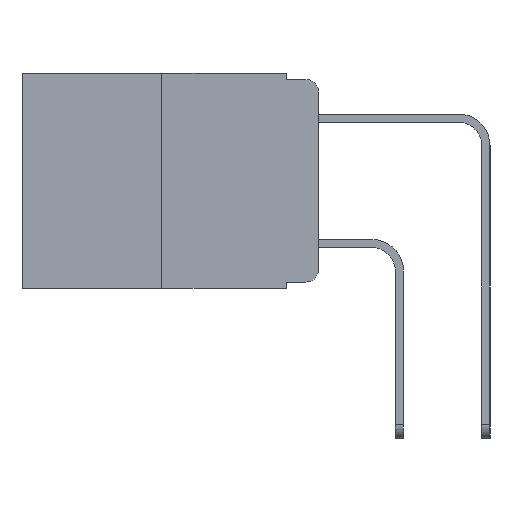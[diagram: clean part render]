
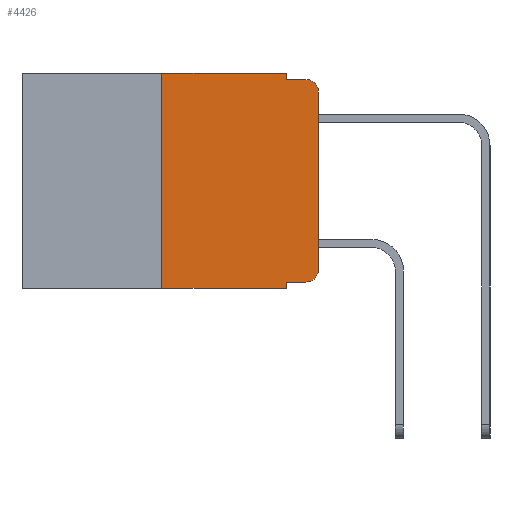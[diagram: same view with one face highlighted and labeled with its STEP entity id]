
A CAD part, left-side view. The second image highlights one B-rep face of the part: STEP entity #4426.
In plain terms, the highlighted planar face has unit normal (-1, 0, 0).
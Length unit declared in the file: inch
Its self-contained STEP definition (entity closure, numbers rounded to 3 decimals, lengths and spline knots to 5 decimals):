
#497 = DIRECTION ( 'NONE',  ( 0., -1., 0. ) ) ;
#598 = CARTESIAN_POINT ( 'NONE',  ( 0., 0.051, -0.333 ) ) ;
#1144 = DIRECTION ( 'NONE',  ( -1., 0., 0. ) ) ;
#1272 = VERTEX_POINT ( 'NONE', #2296 ) ;
#1951 = LINE ( 'NONE', #18520, #19803 ) ;
#2296 = CARTESIAN_POINT ( 'NONE',  ( 0., 0.051, 0. ) ) ;
#2344 = ORIENTED_EDGE ( 'NONE', *, *, #18447, .F. ) ;
#2579 = CARTESIAN_POINT ( 'NONE',  ( 0., 0., -0.313 ) ) ;
#2777 = VERTEX_POINT ( 'NONE', #12425 ) ;
#3322 = CARTESIAN_POINT ( 'NONE',  ( 0., 0.051, 0. ) ) ;
#3454 = CARTESIAN_POINT ( 'NONE',  ( 0., 0.02, -0.01 ) ) ;
#3554 = ORIENTED_EDGE ( 'NONE', *, *, #20716, .T. ) ;
#3621 = CARTESIAN_POINT ( 'NONE',  ( 0., 0.051, -0.333 ) ) ;
#3955 = ORIENTED_EDGE ( 'NONE', *, *, #10687, .F. ) ;
#4123 = CARTESIAN_POINT ( 'NONE',  ( 0., 0.473, -0.343 ) ) ;
#4220 = LINE ( 'NONE', #4123, #22340 ) ;
#4245 = DIRECTION ( 'NONE',  ( 0., 0., -1. ) ) ;
#4426 = ADVANCED_FACE ( 'NONE', ( #16488 ), #11996, .F. ) ;
#4604 = ORIENTED_EDGE ( 'NONE', *, *, #16158, .F. ) ;
#4806 = CARTESIAN_POINT ( 'NONE',  ( 0., 0.25, 0. ) ) ;
#4934 = ORIENTED_EDGE ( 'NONE', *, *, #22171, .T. ) ;
#5609 = ORIENTED_EDGE ( 'NONE', *, *, #14974, .F. ) ;
#5926 = CARTESIAN_POINT ( 'NONE',  ( 0., 0.051, -0.01 ) ) ;
#5939 = CARTESIAN_POINT ( 'NONE',  ( 0., 0., 0. ) ) ;
#5958 = DIRECTION ( 'NONE',  ( 0., -1., 0. ) ) ;
#6283 = VERTEX_POINT ( 'NONE', #3454 ) ;
#6377 = AXIS2_PLACEMENT_3D ( 'NONE', #12093, #1144, #13879 ) ;
#6570 = VERTEX_POINT ( 'NONE', #598 ) ;
#6986 = CARTESIAN_POINT ( 'NONE',  ( 0., 0.25, -0.343 ) ) ;
#7050 = CARTESIAN_POINT ( 'NONE',  ( 0., 0.473, 0. ) ) ;
#7569 = ORIENTED_EDGE ( 'NONE', *, *, #11403, .T. ) ;
#8119 = VECTOR ( 'NONE', #497, 39.37008 ) ;
#8121 = LINE ( 'NONE', #3322, #12861 ) ;
#8598 = CARTESIAN_POINT ( 'NONE',  ( 0., 0.051, -0.01 ) ) ;
#8909 = CARTESIAN_POINT ( 'NONE',  ( 0., 0.051, -0.343 ) ) ;
#10311 = DIRECTION ( 'NONE',  ( 0., 0., 1. ) ) ;
#10410 = LINE ( 'NONE', #3621, #14578 ) ;
#10466 = CARTESIAN_POINT ( 'NONE',  ( 0., 0.473, 0. ) ) ;
#10571 = VERTEX_POINT ( 'NONE', #8598 ) ;
#10687 = EDGE_CURVE ( 'NONE', #18016, #1272, #12916, .T. ) ;
#10804 = CARTESIAN_POINT ( 'NONE',  ( 0., 0.02, -0.313 ) ) ;
#11403 = EDGE_CURVE ( 'NONE', #2777, #19017, #22267, .T. ) ;
#11968 = LINE ( 'NONE', #4806, #16668 ) ;
#11996 = PLANE ( 'NONE',  #13174 ) ;
#12058 = ORIENTED_EDGE ( 'NONE', *, *, #12596, .T. ) ;
#12093 = CARTESIAN_POINT ( 'NONE',  ( 0., 0.02, -0.03 ) ) ;
#12341 = VECTOR ( 'NONE', #16044, 39.37008 ) ;
#12348 = DIRECTION ( 'NONE',  ( 0., 0., -1. ) ) ;
#12425 = CARTESIAN_POINT ( 'NONE',  ( 0., 0.02, -0.333 ) ) ;
#12596 = EDGE_CURVE ( 'NONE', #6570, #2777, #10410, .T. ) ;
#12598 = DIRECTION ( 'NONE',  ( 0., 0., -1. ) ) ;
#12861 = VECTOR ( 'NONE', #12348, 39.37008 ) ;
#12916 = LINE ( 'NONE', #7050, #12341 ) ;
#12924 = AXIS2_PLACEMENT_3D ( 'NONE', #10804, #22858, #12598 ) ;
#13174 = AXIS2_PLACEMENT_3D ( 'NONE', #10466, #22043, #4245 ) ;
#13426 = LINE ( 'NONE', #5926, #8119 ) ;
#13439 = VERTEX_POINT ( 'NONE', #8909 ) ;
#13673 = ORIENTED_EDGE ( 'NONE', *, *, #17315, .T. ) ;
#13784 = EDGE_CURVE ( 'NONE', #6570, #13439, #8121, .T. ) ;
#13790 = CIRCLE ( 'NONE', #6377, 0.02 ) ;
#13879 = DIRECTION ( 'NONE',  ( 0., 0., -1. ) ) ;
#14578 = VECTOR ( 'NONE', #17911, 39.37008 ) ;
#14892 = ORIENTED_EDGE ( 'NONE', *, *, #13784, .F. ) ;
#14974 = EDGE_CURVE ( 'NONE', #17425, #18016, #11968, .T. ) ;
#16044 = DIRECTION ( 'NONE',  ( 0., -1., 0. ) ) ;
#16158 = EDGE_CURVE ( 'NONE', #1272, #10571, #1951, .T. ) ;
#16488 = FACE_OUTER_BOUND ( 'NONE', #22497, .T. ) ;
#16638 = DIRECTION ( 'NONE',  ( 0., 0., 1. ) ) ;
#16668 = VECTOR ( 'NONE', #10311, 39.37008 ) ;
#16870 = VECTOR ( 'NONE', #16638, 39.37008 ) ;
#16878 = DIRECTION ( 'NONE',  ( 0., 0., -1. ) ) ;
#17315 = EDGE_CURVE ( 'NONE', #21411, #6283, #13790, .T. ) ;
#17425 = VERTEX_POINT ( 'NONE', #6986 ) ;
#17911 = DIRECTION ( 'NONE',  ( 0., -1., 0. ) ) ;
#18016 = VERTEX_POINT ( 'NONE', #20925 ) ;
#18447 = EDGE_CURVE ( 'NONE', #10571, #6283, #13426, .T. ) ;
#18520 = CARTESIAN_POINT ( 'NONE',  ( 0., 0.051, 0. ) ) ;
#19017 = VERTEX_POINT ( 'NONE', #2579 ) ;
#19803 = VECTOR ( 'NONE', #16878, 39.37008 ) ;
#20716 = EDGE_CURVE ( 'NONE', #19017, #21411, #21375, .T. ) ;
#20925 = CARTESIAN_POINT ( 'NONE',  ( 0., 0.25, 0. ) ) ;
#21375 = LINE ( 'NONE', #5939, #16870 ) ;
#21411 = VERTEX_POINT ( 'NONE', #22293 ) ;
#22043 = DIRECTION ( 'NONE',  ( 1., 0., 0. ) ) ;
#22171 = EDGE_CURVE ( 'NONE', #17425, #13439, #4220, .T. ) ;
#22267 = CIRCLE ( 'NONE', #12924, 0.02 ) ;
#22293 = CARTESIAN_POINT ( 'NONE',  ( 0., 0., -0.03 ) ) ;
#22340 = VECTOR ( 'NONE', #5958, 39.37008 ) ;
#22497 = EDGE_LOOP ( 'NONE', ( #3554, #13673, #2344, #4604, #3955, #5609, #4934, #14892, #12058, #7569 ) ) ;
#22858 = DIRECTION ( 'NONE',  ( -1., 0., 0. ) ) ;
